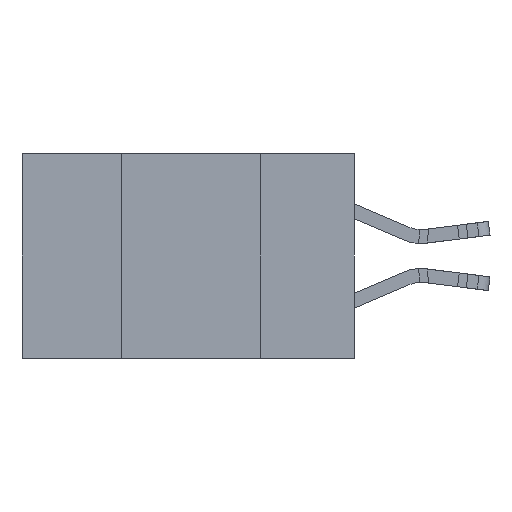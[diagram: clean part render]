
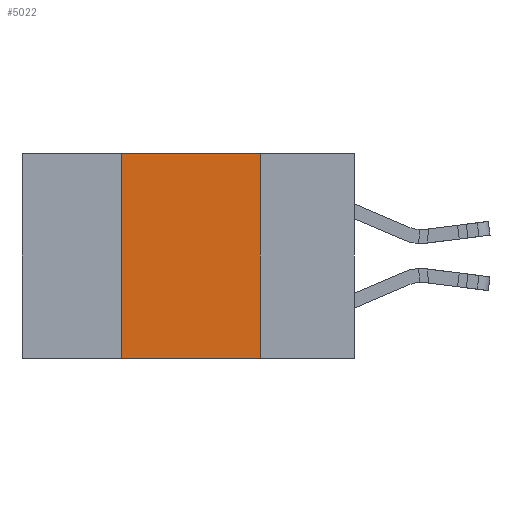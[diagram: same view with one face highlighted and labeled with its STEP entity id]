
A CAD part, left-side view. The second image highlights one B-rep face of the part: STEP entity #5022.
In plain terms, the highlighted planar face has unit normal (-1, 0, 0).
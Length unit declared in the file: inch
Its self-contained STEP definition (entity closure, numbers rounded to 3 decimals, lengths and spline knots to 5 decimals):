
#532 = ORIENTED_EDGE ( 'NONE', *, *, #6844, .T. ) ;
#735 = ORIENTED_EDGE ( 'NONE', *, *, #3229, .F. ) ;
#752 = DIRECTION ( 'NONE',  ( 0., -1., 0. ) ) ;
#1054 = LINE ( 'NONE', #12712, #22331 ) ;
#1258 = ORIENTED_EDGE ( 'NONE', *, *, #19954, .F. ) ;
#1675 = DIRECTION ( 'NONE',  ( 0., 0., -1. ) ) ;
#3011 = LINE ( 'NONE', #8227, #7247 ) ;
#3176 = VERTEX_POINT ( 'NONE', #14490 ) ;
#3229 = EDGE_CURVE ( 'NONE', #19614, #3176, #3011, .T. ) ;
#3790 = CARTESIAN_POINT ( 'NONE',  ( 0., 0.17, 0. ) ) ;
#4988 = VECTOR ( 'NONE', #6490, 39.37008 ) ;
#5022 = ADVANCED_FACE ( 'NONE', ( #17096 ), #6964, .F. ) ;
#6490 = DIRECTION ( 'NONE',  ( 0., 0., -1. ) ) ;
#6844 = EDGE_CURVE ( 'NONE', #19614, #21444, #1054, .T. ) ;
#6964 = PLANE ( 'NONE',  #19479 ) ;
#7247 = VECTOR ( 'NONE', #26728, 39.37008 ) ;
#8099 = ORIENTED_EDGE ( 'NONE', *, *, #33962, .F. ) ;
#8227 = CARTESIAN_POINT ( 'NONE',  ( 0., 0.42, 0. ) ) ;
#12712 = CARTESIAN_POINT ( 'NONE',  ( 0., 0.6, -0.37 ) ) ;
#14490 = CARTESIAN_POINT ( 'NONE',  ( 0., 0.42, 0. ) ) ;
#14972 = CARTESIAN_POINT ( 'NONE',  ( 0., 0.17, 0. ) ) ;
#17096 = FACE_OUTER_BOUND ( 'NONE', #19086, .T. ) ;
#17696 = DIRECTION ( 'NONE',  ( 1., 0., 0. ) ) ;
#18539 = VECTOR ( 'NONE', #752, 39.37008 ) ;
#19086 = EDGE_LOOP ( 'NONE', ( #8099, #1258, #735, #532 ) ) ;
#19339 = CARTESIAN_POINT ( 'NONE',  ( 0., 0.6, 0. ) ) ;
#19479 = AXIS2_PLACEMENT_3D ( 'NONE', #33320, #17696, #1675 ) ;
#19614 = VERTEX_POINT ( 'NONE', #33033 ) ;
#19954 = EDGE_CURVE ( 'NONE', #3176, #32751, #22089, .T. ) ;
#21444 = VERTEX_POINT ( 'NONE', #32699 ) ;
#22089 = LINE ( 'NONE', #19339, #18539 ) ;
#22331 = VECTOR ( 'NONE', #33699, 39.37008 ) ;
#26128 = LINE ( 'NONE', #3790, #4988 ) ;
#26728 = DIRECTION ( 'NONE',  ( 0., 0., 1. ) ) ;
#32699 = CARTESIAN_POINT ( 'NONE',  ( 0., 0.17, -0.37 ) ) ;
#32751 = VERTEX_POINT ( 'NONE', #14972 ) ;
#33033 = CARTESIAN_POINT ( 'NONE',  ( 0., 0.42, -0.37 ) ) ;
#33320 = CARTESIAN_POINT ( 'NONE',  ( 0., 0.6, 0. ) ) ;
#33699 = DIRECTION ( 'NONE',  ( 0., -1., 0. ) ) ;
#33962 = EDGE_CURVE ( 'NONE', #32751, #21444, #26128, .T. ) ;
